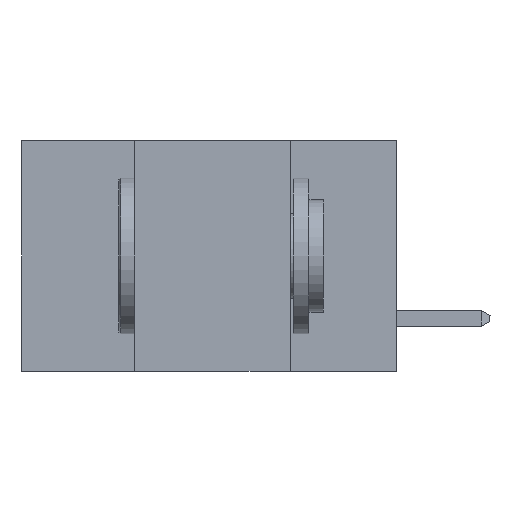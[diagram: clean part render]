
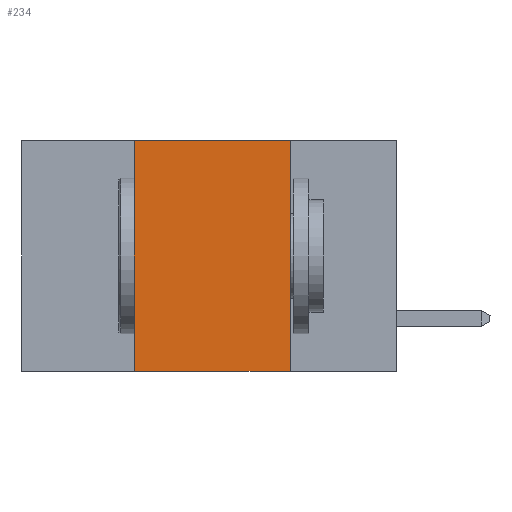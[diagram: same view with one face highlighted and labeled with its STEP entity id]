
A CAD part, left-side view. The second image highlights one B-rep face of the part: STEP entity #234.
In plain terms, the highlighted planar face has unit normal (-1, 0, 0).
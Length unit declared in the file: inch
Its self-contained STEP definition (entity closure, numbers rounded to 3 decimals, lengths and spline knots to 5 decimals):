
#10 = CARTESIAN_POINT ( 'NONE',  ( 0., 0.42, 0. ) ) ;
#132 = CARTESIAN_POINT ( 'NONE',  ( 0., 0.17, 0. ) ) ;
#138 = CARTESIAN_POINT ( 'NONE',  ( 0., 0.6, 0. ) ) ;
#234 = ADVANCED_FACE ( 'NONE', ( #9542 ), #4681, .F. ) ;
#1082 = VERTEX_POINT ( 'NONE', #1619 ) ;
#1314 = LINE ( 'NONE', #10, #5180 ) ;
#1452 = CARTESIAN_POINT ( 'NONE',  ( 0., 0.17, -0.37 ) ) ;
#1466 = VERTEX_POINT ( 'NONE', #2200 ) ;
#1590 = EDGE_CURVE ( 'NONE', #1466, #1082, #1314, .T. ) ;
#1619 = CARTESIAN_POINT ( 'NONE',  ( 0., 0.42, 0. ) ) ;
#1953 = CARTESIAN_POINT ( 'NONE',  ( 0., 0.6, -0.37 ) ) ;
#2099 = LINE ( 'NONE', #1953, #3680 ) ;
#2200 = CARTESIAN_POINT ( 'NONE',  ( 0., 0.42, -0.37 ) ) ;
#2298 = CARTESIAN_POINT ( 'NONE',  ( 0., 0.6, 0. ) ) ;
#2572 = VECTOR ( 'NONE', #6223, 39.37008 ) ;
#3015 = ORIENTED_EDGE ( 'NONE', *, *, #7956, .T. ) ;
#3126 = DIRECTION ( 'NONE',  ( 0., 0., -1. ) ) ;
#3419 = EDGE_CURVE ( 'NONE', #9585, #7802, #5651, .T. ) ;
#3574 = ORIENTED_EDGE ( 'NONE', *, *, #1590, .F. ) ;
#3680 = VECTOR ( 'NONE', #6678, 39.37008 ) ;
#3877 = EDGE_CURVE ( 'NONE', #1082, #9585, #6850, .T. ) ;
#4087 = DIRECTION ( 'NONE',  ( 0., 0., -1. ) ) ;
#4681 = PLANE ( 'NONE',  #6996 ) ;
#5180 = VECTOR ( 'NONE', #5381, 39.37008 ) ;
#5381 = DIRECTION ( 'NONE',  ( 0., 0., 1. ) ) ;
#5651 = LINE ( 'NONE', #132, #6969 ) ;
#6223 = DIRECTION ( 'NONE',  ( 0., -1., 0. ) ) ;
#6610 = ORIENTED_EDGE ( 'NONE', *, *, #3419, .F. ) ;
#6678 = DIRECTION ( 'NONE',  ( 0., -1., 0. ) ) ;
#6850 = LINE ( 'NONE', #2298, #2572 ) ;
#6969 = VECTOR ( 'NONE', #4087, 39.37008 ) ;
#6996 = AXIS2_PLACEMENT_3D ( 'NONE', #138, #7059, #3126 ) ;
#7059 = DIRECTION ( 'NONE',  ( 1., 0., 0. ) ) ;
#7802 = VERTEX_POINT ( 'NONE', #1452 ) ;
#7956 = EDGE_CURVE ( 'NONE', #1466, #7802, #2099, .T. ) ;
#8786 = ORIENTED_EDGE ( 'NONE', *, *, #3877, .F. ) ;
#8883 = EDGE_LOOP ( 'NONE', ( #6610, #8786, #3574, #3015 ) ) ;
#9191 = CARTESIAN_POINT ( 'NONE',  ( 0., 0.17, 0. ) ) ;
#9542 = FACE_OUTER_BOUND ( 'NONE', #8883, .T. ) ;
#9585 = VERTEX_POINT ( 'NONE', #9191 ) ;
